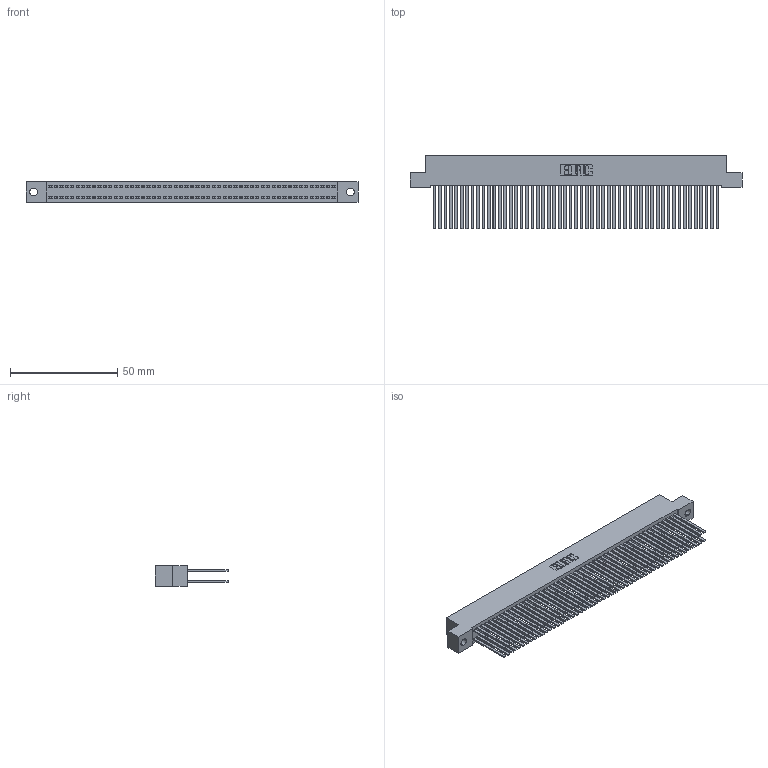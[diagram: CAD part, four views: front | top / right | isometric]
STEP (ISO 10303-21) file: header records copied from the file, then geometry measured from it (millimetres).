
FILE_DESCRIPTION (( 'STEP AP203' ), '1' );
FILE_NAME ('342-106-544-202.STEP', '2018-08-14T07:05:39', ( '' ), ( '' ), 'SwSTEP 2.0', 'SolidWorks 2016', '' );
FILE_SCHEMA (( 'CONFIG_CONTROL_DESIGN' ));
Length unit declared in the file: inch
Products named in the file (3): 342 Part_.128 Slot; 345-292-001_345-293-144; 342-106-544-202
Assembly tree (107 placements, depth 2):
  342-106-544-202
    342 Part_.128 Slot
    345-292-001_345-293-144  x106
Bounding box: 154.94 x 34.3 x 9.4 mm (x, y, z)
Volume: 15407.2 mm3; surface area: 29224.6 mm2
Topology: 107 solids, 107 shells, 4990 faces, 14833 edges, 9746 vertices
Faces by surface type: plane 3462, cylinder 1528
Entity records: 32493 total; most frequent: CARTESIAN_POINT 5370, ORIENTED_EDGE 5306, DIRECTION 4565, EDGE_CURVE 2653, LINE 2529, VECTOR 2529, VERTEX_POINT 1766, AXIS2_PLACEMENT_3D 1018
